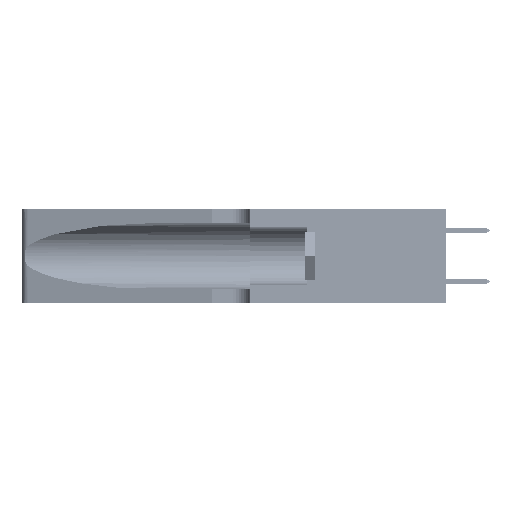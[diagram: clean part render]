
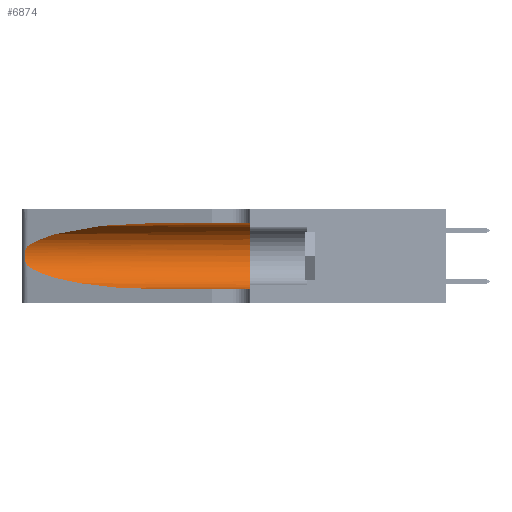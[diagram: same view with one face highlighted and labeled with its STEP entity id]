
A CAD part, left-side view. The second image highlights one B-rep face of the part: STEP entity #6874.
In plain terms, the highlighted cylindrical face has radius 3.308 mm (diameter 6.617 mm), a partial arc.
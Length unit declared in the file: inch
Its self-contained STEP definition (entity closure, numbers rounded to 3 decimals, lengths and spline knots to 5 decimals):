
#668 = ORIENTED_EDGE ( 'NONE', *, *, #772, .T. ) ;
#772 = EDGE_CURVE ( 'NONE', #45968, #14347, #8036, .T. ) ;
#2646 = CARTESIAN_POINT ( 'NONE',  ( 0.1305, 0.72297, 0.05475 ) ) ;
#3402 = DIRECTION ( 'NONE',  ( 0., 0., -1. ) ) ;
#4369 = CIRCLE ( 'NONE', #42317, 0.13025 ) ;
#6426 = CARTESIAN_POINT ( 'NONE',  ( 0.18966, 0.96281, 0.31525 ) ) ;
#6811 = ORIENTED_EDGE ( 'NONE', *, *, #30903, .T. ) ;
#6874 = ADVANCED_FACE ( 'NONE', ( #21809 ), #13247, .F. ) ;
#7303 = VERTEX_POINT ( 'NONE', #24293 ) ;
#8036 =( BOUNDED_CURVE ( )  B_SPLINE_CURVE ( 3, ( #24659, #17152, #9642, #2646 ),
 .UNSPECIFIED., .F., .F. ) 
 B_SPLINE_CURVE_WITH_KNOTS ( ( 4, 4 ),
 ( 3.44316, 4.71239 ),
 .UNSPECIFIED. ) 
 CURVE ( )  GEOMETRIC_REPRESENTATION_ITEM ( )  RATIONAL_B_SPLINE_CURVE ( ( 1., 0.87, 0.87, 1. ) ) 
 REPRESENTATION_ITEM ( '' )  );
#8359 = LINE ( 'NONE', #21794, #44779 ) ;
#9642 = CARTESIAN_POINT ( 'NONE',  ( 0.18966, 0.96281, 0.05475 ) ) ;
#9998 = CARTESIAN_POINT ( 'NONE',  ( 0.1305, 0.35, 0.185 ) ) ;
#10516 = CARTESIAN_POINT ( 'NONE',  ( 0.25555, 1.22994, 0.2215 ) ) ;
#10536 = CARTESIAN_POINT ( 'NONE',  ( 0.25487, 1.22718, 0.22369 ) ) ;
#13247 = CYLINDRICAL_SURFACE ( 'NONE', #19700, 0.13025 ) ;
#13594 = CARTESIAN_POINT ( 'NONE',  ( 0.25555, 1.22993, 0.14849 ) ) ;
#13621 = B_SPLINE_CURVE_WITH_KNOTS ( 'NONE', 3,
 ( #46295, #10516, #35552, #17705, #28698, #35845, #28382, #42804, #32189, #39331, #24614, #36008, #13594, #21394 ),
 .UNSPECIFIED., .F., .F.,
 ( 4, 2, 2, 2, 2, 2, 4 ),
 ( 0., 0.00027, 0.00053, 0.00107, 0.0016, 0.00187, 0.00214 ),
 .UNSPECIFIED. ) ;
#14347 = VERTEX_POINT ( 'NONE', #41841 ) ;
#16662 = VERTEX_POINT ( 'NONE', #23677 ) ;
#17152 = CARTESIAN_POINT ( 'NONE',  ( 0.2373, 1.15595, 0.08982 ) ) ;
#17191 = CARTESIAN_POINT ( 'NONE',  ( 0.1305, 1.61858, 0.05475 ) ) ;
#17705 = CARTESIAN_POINT ( 'NONE',  ( 0.25787, 1.23484, 0.2124 ) ) ;
#17722 = CARTESIAN_POINT ( 'NONE',  ( 0.1305, 0.72297, 0.31525 ) ) ;
#19700 = AXIS2_PLACEMENT_3D ( 'NONE', #43130, #39360, #3402 ) ;
#20129 = LINE ( 'NONE', #17191, #25809 ) ;
#21394 = CARTESIAN_POINT ( 'NONE',  ( 0.25487, 1.22718, 0.14631 ) ) ;
#21794 = CARTESIAN_POINT ( 'NONE',  ( 0.1305, 1.61858, 0.31525 ) ) ;
#21809 = FACE_OUTER_BOUND ( 'NONE', #34228, .T. ) ;
#22897 = ORIENTED_EDGE ( 'NONE', *, *, #34345, .F. ) ;
#23677 = CARTESIAN_POINT ( 'NONE',  ( 0.1305, 0.35, 0.31525 ) ) ;
#24077 = ORIENTED_EDGE ( 'NONE', *, *, #32582, .T. ) ;
#24293 = CARTESIAN_POINT ( 'NONE',  ( 0.1305, 0.35, 0.05475 ) ) ;
#24614 = CARTESIAN_POINT ( 'NONE',  ( 0.25789, 1.23486, 0.15765 ) ) ;
#24659 = CARTESIAN_POINT ( 'NONE',  ( 0.25487, 1.22718, 0.14631 ) ) ;
#24839 = DIRECTION ( 'NONE',  ( 0., -1., 0. ) ) ;
#24970 = CARTESIAN_POINT ( 'NONE',  ( 0.1305, 0.72297, 0.31525 ) ) ;
#24991 = CARTESIAN_POINT ( 'NONE',  ( 0.25487, 1.22718, 0.22369 ) ) ;
#25004 = DIRECTION ( 'NONE',  ( 0., -1., 0. ) ) ;
#25809 = VECTOR ( 'NONE', #25004, 39.37008 ) ;
#28026 = DIRECTION ( 'NONE',  ( 0., 0., 1. ) ) ;
#28382 = CARTESIAN_POINT ( 'NONE',  ( 0.26075, 1.23896, 0.19203 ) ) ;
#28698 = CARTESIAN_POINT ( 'NONE',  ( 0.25854, 1.2359, 0.20912 ) ) ;
#29090 =( BOUNDED_CURVE ( )  B_SPLINE_CURVE ( 3, ( #17722, #6426, #32053, #10536 ),
 .UNSPECIFIED., .F., .T. ) 
 B_SPLINE_CURVE_WITH_KNOTS ( ( 4, 4 ),
 ( 1.5708, 2.84003 ),
 .UNSPECIFIED. ) 
 CURVE ( )  GEOMETRIC_REPRESENTATION_ITEM ( )  RATIONAL_B_SPLINE_CURVE ( ( 1., 0.87, 0.87, 1. ) ) 
 REPRESENTATION_ITEM ( '' )  );
#30295 = VERTEX_POINT ( 'NONE', #24970 ) ;
#30903 = EDGE_CURVE ( 'NONE', #30295, #43116, #29090, .T. ) ;
#32053 = CARTESIAN_POINT ( 'NONE',  ( 0.2373, 1.15595, 0.28018 ) ) ;
#32189 = CARTESIAN_POINT ( 'NONE',  ( 0.26017, 1.23833, 0.17102 ) ) ;
#32582 = EDGE_CURVE ( 'NONE', #14347, #7303, #20129, .T. ) ;
#33819 = ORIENTED_EDGE ( 'NONE', *, *, #42973, .F. ) ;
#34228 = EDGE_LOOP ( 'NONE', ( #6811, #41490, #668, #24077, #22897, #33819 ) ) ;
#34345 = EDGE_CURVE ( 'NONE', #16662, #7303, #4369, .T. ) ;
#34944 = CARTESIAN_POINT ( 'NONE',  ( 0.25487, 1.22718, 0.14631 ) ) ;
#35552 = CARTESIAN_POINT ( 'NONE',  ( 0.25639, 1.23184, 0.21858 ) ) ;
#35845 = CARTESIAN_POINT ( 'NONE',  ( 0.26018, 1.23835, 0.19895 ) ) ;
#36008 = CARTESIAN_POINT ( 'NONE',  ( 0.25639, 1.23186, 0.15144 ) ) ;
#38274 = EDGE_CURVE ( 'NONE', #43116, #45968, #13621, .T. ) ;
#39331 = CARTESIAN_POINT ( 'NONE',  ( 0.25856, 1.23593, 0.16098 ) ) ;
#39360 = DIRECTION ( 'NONE',  ( 0., -1., 0. ) ) ;
#41490 = ORIENTED_EDGE ( 'NONE', *, *, #38274, .T. ) ;
#41841 = CARTESIAN_POINT ( 'NONE',  ( 0.1305, 0.72297, 0.05475 ) ) ;
#42317 = AXIS2_PLACEMENT_3D ( 'NONE', #9998, #46533, #28026 ) ;
#42804 = CARTESIAN_POINT ( 'NONE',  ( 0.26075, 1.23896, 0.178 ) ) ;
#42973 = EDGE_CURVE ( 'NONE', #30295, #16662, #8359, .T. ) ;
#43116 = VERTEX_POINT ( 'NONE', #24991 ) ;
#43130 = CARTESIAN_POINT ( 'NONE',  ( 0.1305, 1.61858, 0.185 ) ) ;
#44779 = VECTOR ( 'NONE', #24839, 39.37008 ) ;
#45968 = VERTEX_POINT ( 'NONE', #34944 ) ;
#46295 = CARTESIAN_POINT ( 'NONE',  ( 0.25487, 1.22718, 0.22369 ) ) ;
#46533 = DIRECTION ( 'NONE',  ( 0., 1., 0. ) ) ;
